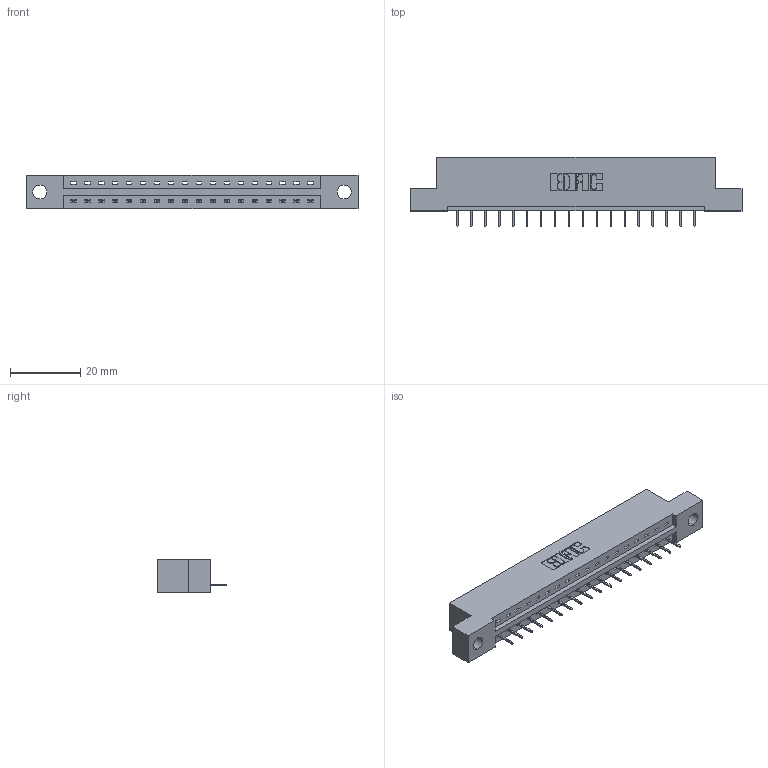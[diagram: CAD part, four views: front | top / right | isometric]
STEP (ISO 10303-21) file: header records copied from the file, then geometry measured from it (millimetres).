
FILE_DESCRIPTION (( 'STEP AP203' ), '1' );
FILE_NAME ('387-018-524-104.STEP', '2019-10-02T20:08:14', ( '' ), ( '' ), 'SwSTEP 2.0', 'SolidWorks 2016', '' );
FILE_SCHEMA (( 'CONFIG_CONTROL_DESIGN' ));
Length unit declared in the file: inch
Products named in the file (3): 387-018-524-104; 337 Part_Flush Mounting Lugs - 0.156 Dia-TH; 345-292-001_345-293-124
Assembly tree (19 placements, depth 2):
  387-018-524-104
    337 Part_Flush Mounting Lugs - 0.156 Dia-TH
    345-292-001_345-293-124  x18
Bounding box: 94.34 x 19.69 x 9.4 mm (x, y, z)
Volume: 9345.3 mm3; surface area: 9069 mm2
Topology: 19 solids, 19 shells, 1302 faces, 3767 edges, 2438 vertices
Faces by surface type: plane 1006, cylinder 296
Entity records: 16561 total; most frequent: CARTESIAN_POINT 2888, ORIENTED_EDGE 2842, DIRECTION 2481, EDGE_CURVE 1421, LINE 1297, VECTOR 1297, VERTEX_POINT 942, AXIS2_PLACEMENT_3D 592
